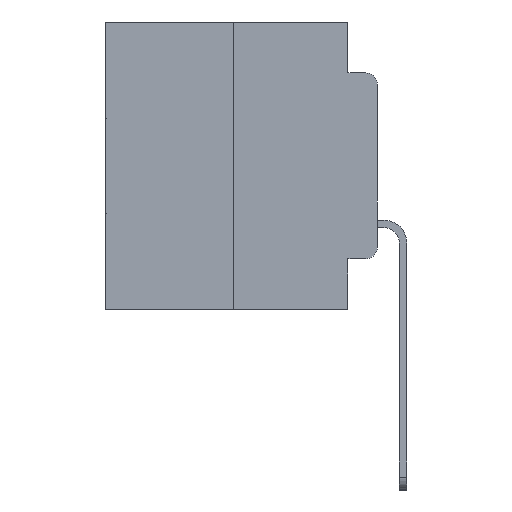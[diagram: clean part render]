
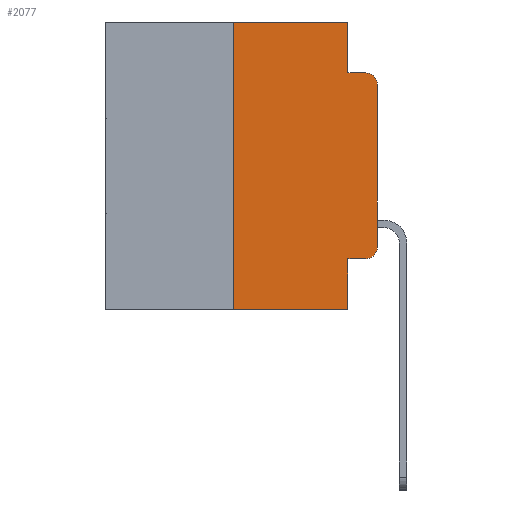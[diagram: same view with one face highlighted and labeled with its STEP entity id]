
A CAD part, left-side view. The second image highlights one B-rep face of the part: STEP entity #2077.
In plain terms, the highlighted planar face has unit normal (-1, 0, 0).
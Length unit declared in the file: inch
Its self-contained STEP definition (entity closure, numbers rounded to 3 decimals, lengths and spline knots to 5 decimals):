
#419 = EDGE_CURVE ( 'NONE', #28159, #6516, #19290, .T. ) ;
#679 = VERTEX_POINT ( 'NONE', #13951 ) ;
#901 = CARTESIAN_POINT ( 'NONE',  ( 0., 0.473, -0.5 ) ) ;
#1445 = CIRCLE ( 'NONE', #19039, 0.02 ) ;
#1953 = ORIENTED_EDGE ( 'NONE', *, *, #7445, .T. ) ;
#2029 = DIRECTION ( 'NONE',  ( 0., 0., -1. ) ) ;
#2077 = ADVANCED_FACE ( 'NONE', ( #24079 ), #14651, .F. ) ;
#2514 = CARTESIAN_POINT ( 'NONE',  ( 0., 0.051, -0.4115 ) ) ;
#2658 = EDGE_CURVE ( 'NONE', #19978, #15999, #13562, .T. ) ;
#2822 = EDGE_CURVE ( 'NONE', #15999, #25113, #19155, .T. ) ;
#3273 = LINE ( 'NONE', #16675, #25171 ) ;
#3646 = VECTOR ( 'NONE', #25070, 39.37008 ) ;
#4128 = CARTESIAN_POINT ( 'NONE',  ( 0., 0.25, 0. ) ) ;
#4200 = CARTESIAN_POINT ( 'NONE',  ( 0., 0.051, 0. ) ) ;
#5232 = EDGE_CURVE ( 'NONE', #19978, #7381, #12294, .T. ) ;
#5621 = DIRECTION ( 'NONE',  ( 0., 0., 1. ) ) ;
#5917 = CARTESIAN_POINT ( 'NONE',  ( 0., 0.02, -0.1085 ) ) ;
#6151 = DIRECTION ( 'NONE',  ( 0., 0., -1. ) ) ;
#6342 = CARTESIAN_POINT ( 'NONE',  ( 0., 0., -0.3915 ) ) ;
#6516 = VERTEX_POINT ( 'NONE', #8027 ) ;
#6614 = CARTESIAN_POINT ( 'NONE',  ( 0., 0.473, 0. ) ) ;
#7381 = VERTEX_POINT ( 'NONE', #15991 ) ;
#7445 = EDGE_CURVE ( 'NONE', #23264, #679, #1445, .T. ) ;
#8027 = CARTESIAN_POINT ( 'NONE',  ( 0., 0.25, 0. ) ) ;
#8075 = CARTESIAN_POINT ( 'NONE',  ( 0., 0., -0.1085 ) ) ;
#8126 = DIRECTION ( 'NONE',  ( 0., 0., -1. ) ) ;
#8139 = VERTEX_POINT ( 'NONE', #4200 ) ;
#8631 = ORIENTED_EDGE ( 'NONE', *, *, #5232, .F. ) ;
#9788 = CARTESIAN_POINT ( 'NONE',  ( 0., 0.051, 0. ) ) ;
#10071 = DIRECTION ( 'NONE',  ( 0., -1., 0. ) ) ;
#10476 = CARTESIAN_POINT ( 'NONE',  ( 0., 0.02, -0.3915 ) ) ;
#10934 = VECTOR ( 'NONE', #19987, 39.37008 ) ;
#12249 = CARTESIAN_POINT ( 'NONE',  ( 0., 0.051, -0.0885 ) ) ;
#12294 = LINE ( 'NONE', #25179, #3646 ) ;
#12406 = LINE ( 'NONE', #27835, #26009 ) ;
#12992 = AXIS2_PLACEMENT_3D ( 'NONE', #10476, #14930, #2029 ) ;
#13069 = CARTESIAN_POINT ( 'NONE',  ( 0., 0.25, -0.5 ) ) ;
#13562 = LINE ( 'NONE', #2514, #22277 ) ;
#13883 = EDGE_CURVE ( 'NONE', #8139, #19939, #23216, .T. ) ;
#13951 = CARTESIAN_POINT ( 'NONE',  ( 0., 0.02, -0.0885 ) ) ;
#14329 = DIRECTION ( 'NONE',  ( 0., -1., 0. ) ) ;
#14651 = PLANE ( 'NONE',  #19134 ) ;
#14807 = DIRECTION ( 'NONE',  ( -1., 0., 0. ) ) ;
#14930 = DIRECTION ( 'NONE',  ( -1., 0., 0. ) ) ;
#15078 = LINE ( 'NONE', #901, #26216 ) ;
#15251 = DIRECTION ( 'NONE',  ( 0., 0., 1. ) ) ;
#15279 = ORIENTED_EDGE ( 'NONE', *, *, #13883, .F. ) ;
#15991 = CARTESIAN_POINT ( 'NONE',  ( 0., 0.051, -0.5 ) ) ;
#15999 = VERTEX_POINT ( 'NONE', #21111 ) ;
#16268 = ORIENTED_EDGE ( 'NONE', *, *, #419, .F. ) ;
#16641 = ORIENTED_EDGE ( 'NONE', *, *, #2658, .T. ) ;
#16675 = CARTESIAN_POINT ( 'NONE',  ( 0., 0., 0. ) ) ;
#17188 = ORIENTED_EDGE ( 'NONE', *, *, #28531, .T. ) ;
#17212 = LINE ( 'NONE', #6614, #10934 ) ;
#17738 = EDGE_CURVE ( 'NONE', #19939, #679, #12406, .T. ) ;
#18280 = EDGE_LOOP ( 'NONE', ( #27036, #1953, #27749, #15279, #25952, #16268, #17188, #8631, #16641, #23653 ) ) ;
#18676 = VECTOR ( 'NONE', #23191, 39.37008 ) ;
#19039 = AXIS2_PLACEMENT_3D ( 'NONE', #5917, #14807, #8126 ) ;
#19130 = DIRECTION ( 'NONE',  ( 1., 0., 0. ) ) ;
#19134 = AXIS2_PLACEMENT_3D ( 'NONE', #19416, #19130, #6151 ) ;
#19155 = CIRCLE ( 'NONE', #12992, 0.02 ) ;
#19290 = LINE ( 'NONE', #4128, #20312 ) ;
#19416 = CARTESIAN_POINT ( 'NONE',  ( 0., 0.473, 0. ) ) ;
#19939 = VERTEX_POINT ( 'NONE', #12249 ) ;
#19978 = VERTEX_POINT ( 'NONE', #27629 ) ;
#19987 = DIRECTION ( 'NONE',  ( 0., -1., 0. ) ) ;
#20312 = VECTOR ( 'NONE', #15251, 39.37008 ) ;
#21111 = CARTESIAN_POINT ( 'NONE',  ( 0., 0.02, -0.4115 ) ) ;
#22277 = VECTOR ( 'NONE', #27394, 39.37008 ) ;
#23191 = DIRECTION ( 'NONE',  ( 0., 0., -1. ) ) ;
#23216 = LINE ( 'NONE', #9788, #18676 ) ;
#23264 = VERTEX_POINT ( 'NONE', #8075 ) ;
#23653 = ORIENTED_EDGE ( 'NONE', *, *, #2822, .T. ) ;
#24079 = FACE_OUTER_BOUND ( 'NONE', #18280, .T. ) ;
#25070 = DIRECTION ( 'NONE',  ( 0., 0., -1. ) ) ;
#25113 = VERTEX_POINT ( 'NONE', #6342 ) ;
#25171 = VECTOR ( 'NONE', #5621, 39.37008 ) ;
#25179 = CARTESIAN_POINT ( 'NONE',  ( 0., 0.051, 0. ) ) ;
#25952 = ORIENTED_EDGE ( 'NONE', *, *, #28195, .F. ) ;
#26009 = VECTOR ( 'NONE', #10071, 39.37008 ) ;
#26216 = VECTOR ( 'NONE', #14329, 39.37008 ) ;
#27036 = ORIENTED_EDGE ( 'NONE', *, *, #28548, .T. ) ;
#27394 = DIRECTION ( 'NONE',  ( 0., -1., 0. ) ) ;
#27629 = CARTESIAN_POINT ( 'NONE',  ( 0., 0.051, -0.4115 ) ) ;
#27749 = ORIENTED_EDGE ( 'NONE', *, *, #17738, .F. ) ;
#27835 = CARTESIAN_POINT ( 'NONE',  ( 0., 0.051, -0.0885 ) ) ;
#28159 = VERTEX_POINT ( 'NONE', #13069 ) ;
#28195 = EDGE_CURVE ( 'NONE', #6516, #8139, #17212, .T. ) ;
#28531 = EDGE_CURVE ( 'NONE', #28159, #7381, #15078, .T. ) ;
#28548 = EDGE_CURVE ( 'NONE', #25113, #23264, #3273, .T. ) ;
